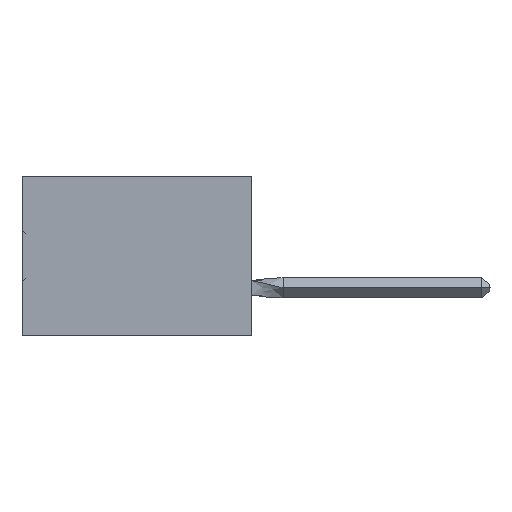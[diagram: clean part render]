
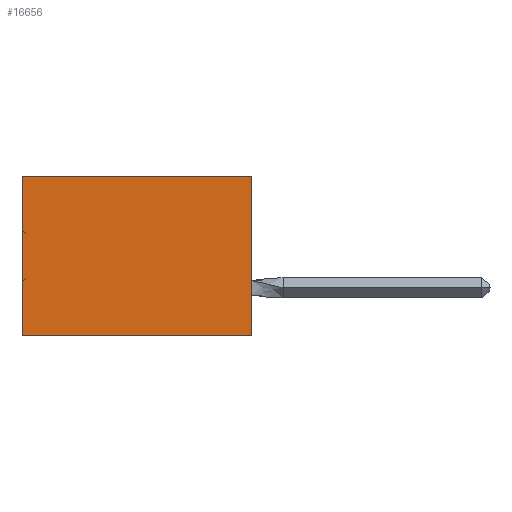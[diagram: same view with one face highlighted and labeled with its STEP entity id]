
A CAD part, left-side view. The second image highlights one B-rep face of the part: STEP entity #16656.
In plain terms, the highlighted planar face has unit normal (-1, 0, 0).
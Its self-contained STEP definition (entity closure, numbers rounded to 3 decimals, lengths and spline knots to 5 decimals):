
#1127 = PLANE ( 'NONE',  #31487 ) ;
#1321 = CARTESIAN_POINT ( 'NONE',  ( 0.305, 0., -0.5 ) ) ;
#2685 = EDGE_CURVE ( 'NONE', #41740, #5230, #43727, .T. ) ;
#2858 = FACE_OUTER_BOUND ( 'NONE', #20544, .T. ) ;
#3626 = VECTOR ( 'NONE', #53115, 39.37008 ) ;
#5230 = VERTEX_POINT ( 'NONE', #11705 ) ;
#6244 = CARTESIAN_POINT ( 'NONE',  ( 0.305, 0., 0. ) ) ;
#9050 = DIRECTION ( 'NONE',  ( 0., 1., 0. ) ) ;
#10456 = VECTOR ( 'NONE', #14807, 39.37008 ) ;
#10464 = DIRECTION ( 'NONE',  ( 1., 0., 0. ) ) ;
#11705 = CARTESIAN_POINT ( 'NONE',  ( 0.305, 0.72, 0. ) ) ;
#13126 = EDGE_CURVE ( 'NONE', #41740, #16717, #35319, .T. ) ;
#14787 = VECTOR ( 'NONE', #41521, 39.37008 ) ;
#14807 = DIRECTION ( 'NONE',  ( 0., 0., -1. ) ) ;
#15553 = LINE ( 'NONE', #17662, #14787 ) ;
#16656 = ADVANCED_FACE ( 'NONE', ( #2858 ), #1127, .F. ) ;
#16717 = VERTEX_POINT ( 'NONE', #32745 ) ;
#17662 = CARTESIAN_POINT ( 'NONE',  ( 0.305, 0.72, -0.5 ) ) ;
#19679 = VERTEX_POINT ( 'NONE', #45572 ) ;
#19720 = EDGE_CURVE ( 'NONE', #16717, #19679, #27358, .T. ) ;
#20544 = EDGE_LOOP ( 'NONE', ( #43737, #48943, #60039, #35952 ) ) ;
#23838 = CARTESIAN_POINT ( 'NONE',  ( 0.305, 0., -0.5 ) ) ;
#27358 = LINE ( 'NONE', #32137, #28801 ) ;
#28801 = VECTOR ( 'NONE', #9050, 39.37008 ) ;
#31487 = AXIS2_PLACEMENT_3D ( 'NONE', #1321, #10464, #43117 ) ;
#32137 = CARTESIAN_POINT ( 'NONE',  ( 0.305, 0., -0.5 ) ) ;
#32745 = CARTESIAN_POINT ( 'NONE',  ( 0.305, 0., -0.5 ) ) ;
#35319 = LINE ( 'NONE', #23838, #10456 ) ;
#35684 = EDGE_CURVE ( 'NONE', #5230, #19679, #15553, .T. ) ;
#35952 = ORIENTED_EDGE ( 'NONE', *, *, #2685, .T. ) ;
#41521 = DIRECTION ( 'NONE',  ( 0., 0., -1. ) ) ;
#41740 = VERTEX_POINT ( 'NONE', #46918 ) ;
#43117 = DIRECTION ( 'NONE',  ( 0., 0., -1. ) ) ;
#43727 = LINE ( 'NONE', #6244, #3626 ) ;
#43737 = ORIENTED_EDGE ( 'NONE', *, *, #35684, .T. ) ;
#45572 = CARTESIAN_POINT ( 'NONE',  ( 0.305, 0.72, -0.5 ) ) ;
#46918 = CARTESIAN_POINT ( 'NONE',  ( 0.305, 0., 0. ) ) ;
#48943 = ORIENTED_EDGE ( 'NONE', *, *, #19720, .F. ) ;
#53115 = DIRECTION ( 'NONE',  ( 0., 1., 0. ) ) ;
#60039 = ORIENTED_EDGE ( 'NONE', *, *, #13126, .F. ) ;
